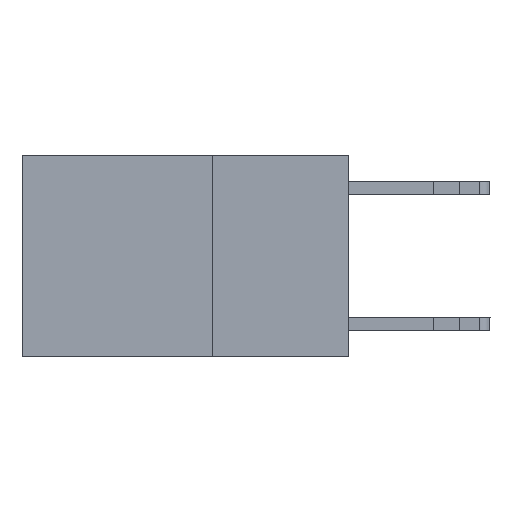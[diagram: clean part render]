
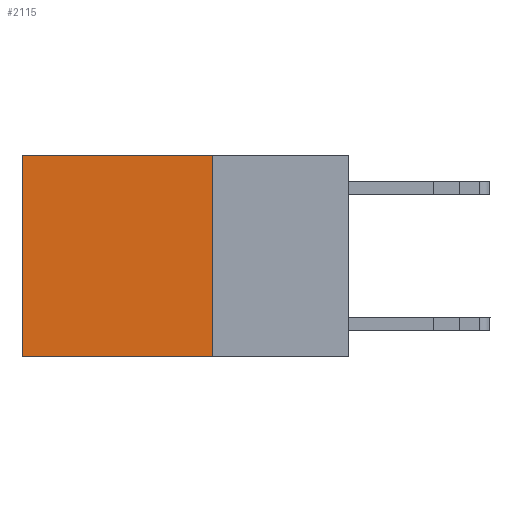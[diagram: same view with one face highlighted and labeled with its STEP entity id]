
A CAD part, left-side view. The second image highlights one B-rep face of the part: STEP entity #2115.
In plain terms, the highlighted planar face has unit normal (-1, 0, 0).
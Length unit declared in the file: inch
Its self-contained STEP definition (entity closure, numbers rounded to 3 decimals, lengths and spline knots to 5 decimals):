
#601 = EDGE_CURVE ( 'NONE', #10442, #11980, #1264, .T. ) ;
#1227 = VECTOR ( 'NONE', #4114, 39.37008 ) ;
#1264 = LINE ( 'NONE', #21878, #1227 ) ;
#2115 = ADVANCED_FACE ( 'NONE', ( #16252 ), #13009, .F. ) ;
#2861 = EDGE_CURVE ( 'NONE', #24100, #11980, #8072, .T. ) ;
#4114 = DIRECTION ( 'NONE',  ( 0., 1., 0. ) ) ;
#4330 = ORIENTED_EDGE ( 'NONE', *, *, #14002, .T. ) ;
#6044 = DIRECTION ( 'NONE',  ( 0., 0., -1. ) ) ;
#6181 = DIRECTION ( 'NONE',  ( 0., 1., 0. ) ) ;
#6221 = CARTESIAN_POINT ( 'NONE',  ( 0.2625, 0.25, 0. ) ) ;
#8072 = LINE ( 'NONE', #12038, #8146 ) ;
#8146 = VECTOR ( 'NONE', #10283, 39.37008 ) ;
#8932 = CARTESIAN_POINT ( 'NONE',  ( 0.2625, 0.6, -0.37 ) ) ;
#9353 = AXIS2_PLACEMENT_3D ( 'NONE', #12724, #12671, #12584 ) ;
#9912 = EDGE_LOOP ( 'NONE', ( #20900, #19883, #25987, #4330 ) ) ;
#10283 = DIRECTION ( 'NONE',  ( 0., 0., -1. ) ) ;
#10442 = VERTEX_POINT ( 'NONE', #17162 ) ;
#10896 = LINE ( 'NONE', #6221, #11018 ) ;
#11018 = VECTOR ( 'NONE', #6181, 39.37008 ) ;
#11798 = CARTESIAN_POINT ( 'NONE',  ( 0.2625, 0.6, 0. ) ) ;
#11980 = VERTEX_POINT ( 'NONE', #8932 ) ;
#12038 = CARTESIAN_POINT ( 'NONE',  ( 0.2625, 0.6, 0. ) ) ;
#12584 = DIRECTION ( 'NONE',  ( 0., 0., -1. ) ) ;
#12671 = DIRECTION ( 'NONE',  ( 1., 0., 0. ) ) ;
#12724 = CARTESIAN_POINT ( 'NONE',  ( 0.2625, 0.25, 0. ) ) ;
#13009 = PLANE ( 'NONE',  #9353 ) ;
#14002 = EDGE_CURVE ( 'NONE', #20676, #24100, #10896, .T. ) ;
#16252 = FACE_OUTER_BOUND ( 'NONE', #9912, .T. ) ;
#17162 = CARTESIAN_POINT ( 'NONE',  ( 0.2625, 0.25, -0.37 ) ) ;
#19883 = ORIENTED_EDGE ( 'NONE', *, *, #601, .F. ) ;
#20142 = CARTESIAN_POINT ( 'NONE',  ( 0.2625, 0.25, 0. ) ) ;
#20534 = CARTESIAN_POINT ( 'NONE',  ( 0.2625, 0.25, 0. ) ) ;
#20676 = VERTEX_POINT ( 'NONE', #20142 ) ;
#20900 = ORIENTED_EDGE ( 'NONE', *, *, #2861, .T. ) ;
#21878 = CARTESIAN_POINT ( 'NONE',  ( 0.2625, 0.25, -0.37 ) ) ;
#24100 = VERTEX_POINT ( 'NONE', #11798 ) ;
#25860 = VECTOR ( 'NONE', #6044, 39.37008 ) ;
#25987 = ORIENTED_EDGE ( 'NONE', *, *, #26664, .F. ) ;
#26073 = LINE ( 'NONE', #20534, #25860 ) ;
#26664 = EDGE_CURVE ( 'NONE', #20676, #10442, #26073, .T. ) ;
